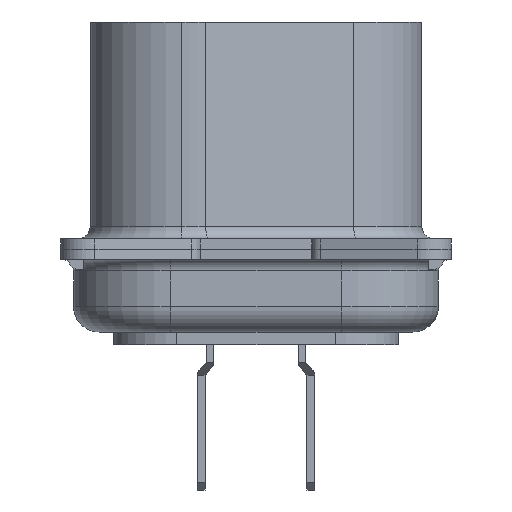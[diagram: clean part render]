
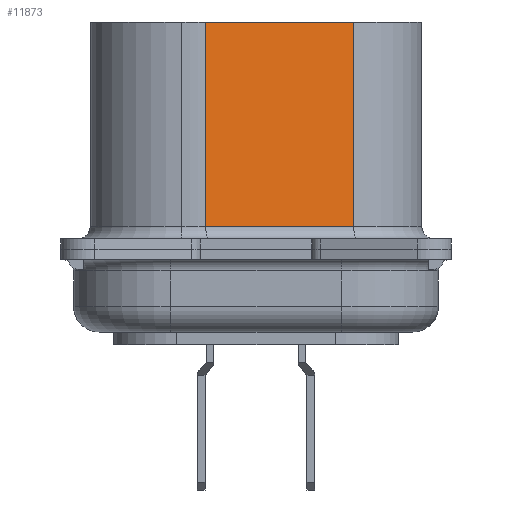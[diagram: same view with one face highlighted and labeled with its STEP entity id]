
A CAD part, left-side view. The second image highlights one B-rep face of the part: STEP entity #11873.
In plain terms, the highlighted planar face has unit normal (-0.966, -0.259, 0).
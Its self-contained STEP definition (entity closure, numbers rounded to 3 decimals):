
#2171 = CARTESIAN_POINT ( 'NONE',  ( 6.467, -3.832, 9.3 ) ) ;
#2182 = ORIENTED_EDGE ( 'NONE', *, *, #64242, .F. ) ;
#7705 = VERTEX_POINT ( 'NONE', #48947 ) ;
#11873 = ADVANCED_FACE ( 'NONE', ( #109183 ), #107615, .F. ) ;
#14852 = CARTESIAN_POINT ( 'NONE',  ( 6.467, -3.832, 9.3 ) ) ;
#24191 = DIRECTION ( 'NONE',  ( -0.259, 0.966, 0. ) ) ;
#24970 = DIRECTION ( 'NONE',  ( 0.966, 0.259, 0. ) ) ;
#28439 = CARTESIAN_POINT ( 'NONE',  ( 6.467, -3.832, 1.3 ) ) ;
#31560 = EDGE_CURVE ( 'NONE', #133777, #136449, #63025, .T. ) ;
#34714 = AXIS2_PLACEMENT_3D ( 'NONE', #2171, #24970, #24191 ) ;
#42254 = VECTOR ( 'NONE', #151116, 1000. ) ;
#46642 = CARTESIAN_POINT ( 'NONE',  ( 4.913, 1.968, 9.3 ) ) ;
#48947 = CARTESIAN_POINT ( 'NONE',  ( 4.913, 1.968, 1.3 ) ) ;
#51255 = DIRECTION ( 'NONE',  ( 0.259, -0.966, 0. ) ) ;
#56368 = LINE ( 'NONE', #150767, #78177 ) ;
#57125 = LINE ( 'NONE', #104378, #80516 ) ;
#63025 = LINE ( 'NONE', #74097, #96852 ) ;
#64242 = EDGE_CURVE ( 'NONE', #136449, #149268, #57125, .T. ) ;
#68955 = CARTESIAN_POINT ( 'NONE',  ( 6.467, -3.832, 1.3 ) ) ;
#74097 = CARTESIAN_POINT ( 'NONE',  ( 6.467, -3.832, 9.3 ) ) ;
#74116 = ORIENTED_EDGE ( 'NONE', *, *, #100130, .T. ) ;
#74701 = ORIENTED_EDGE ( 'NONE', *, *, #31560, .F. ) ;
#78177 = VECTOR ( 'NONE', #127935, 1000. ) ;
#80516 = VECTOR ( 'NONE', #80725, 1000. ) ;
#80725 = DIRECTION ( 'NONE',  ( 0., 0., -1. ) ) ;
#89430 = ORIENTED_EDGE ( 'NONE', *, *, #122857, .T. ) ;
#91212 = EDGE_LOOP ( 'NONE', ( #89430, #74116, #2182, #74701 ) ) ;
#96852 = VECTOR ( 'NONE', #51255, 1000. ) ;
#100130 = EDGE_CURVE ( 'NONE', #7705, #149268, #101612, .T. ) ;
#101612 = LINE ( 'NONE', #28439, #42254 ) ;
#104378 = CARTESIAN_POINT ( 'NONE',  ( 6.467, -3.832, 9.3 ) ) ;
#107615 = PLANE ( 'NONE',  #34714 ) ;
#109183 = FACE_OUTER_BOUND ( 'NONE', #91212, .T. ) ;
#122857 = EDGE_CURVE ( 'NONE', #133777, #7705, #56368, .T. ) ;
#127935 = DIRECTION ( 'NONE',  ( 0., 0., -1. ) ) ;
#133777 = VERTEX_POINT ( 'NONE', #46642 ) ;
#136449 = VERTEX_POINT ( 'NONE', #14852 ) ;
#149268 = VERTEX_POINT ( 'NONE', #68955 ) ;
#150767 = CARTESIAN_POINT ( 'NONE',  ( 4.913, 1.968, 9.3 ) ) ;
#151116 = DIRECTION ( 'NONE',  ( 0.259, -0.966, 0. ) ) ;
